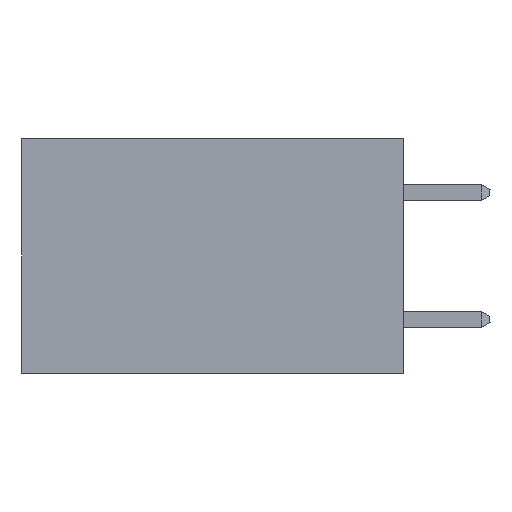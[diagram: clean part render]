
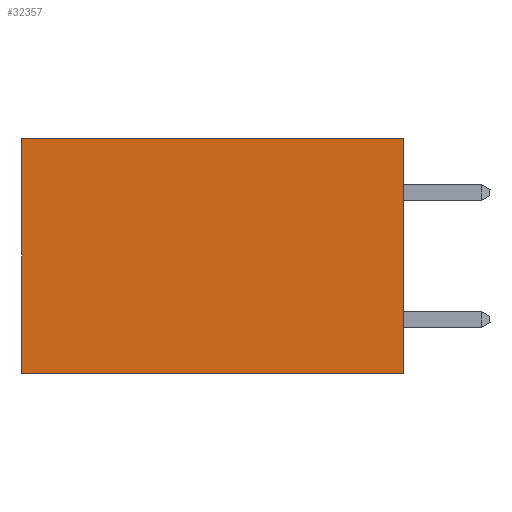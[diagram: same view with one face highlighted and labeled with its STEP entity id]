
A CAD part, left-side view. The second image highlights one B-rep face of the part: STEP entity #32357.
In plain terms, the highlighted planar face has unit normal (-1, 0, 0).
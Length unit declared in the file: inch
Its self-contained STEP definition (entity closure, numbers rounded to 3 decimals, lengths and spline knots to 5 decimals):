
#1623 = CARTESIAN_POINT ( 'NONE',  ( 0.2875, 0., 0. ) ) ;
#1764 = VERTEX_POINT ( 'NONE', #30921 ) ;
#2161 = DIRECTION ( 'NONE',  ( 0., 0., -1. ) ) ;
#2675 = LINE ( 'NONE', #16467, #3827 ) ;
#3013 = PLANE ( 'NONE',  #22933 ) ;
#3535 = ORIENTED_EDGE ( 'NONE', *, *, #15642, .F. ) ;
#3827 = VECTOR ( 'NONE', #2161, 39.37008 ) ;
#7677 = VECTOR ( 'NONE', #17593, 39.37008 ) ;
#7687 = DIRECTION ( 'NONE',  ( 0., 0., -1. ) ) ;
#8514 = FACE_OUTER_BOUND ( 'NONE', #14511, .T. ) ;
#9731 = LINE ( 'NONE', #27854, #22397 ) ;
#10199 = LINE ( 'NONE', #27157, #28822 ) ;
#13163 = ORIENTED_EDGE ( 'NONE', *, *, #20071, .T. ) ;
#14511 = EDGE_LOOP ( 'NONE', ( #13163, #3535, #28302, #31554 ) ) ;
#15642 = EDGE_CURVE ( 'NONE', #30937, #1764, #16727, .T. ) ;
#16467 = CARTESIAN_POINT ( 'NONE',  ( 0.2875, 0.6, 0. ) ) ;
#16727 = LINE ( 'NONE', #27665, #7677 ) ;
#17593 = DIRECTION ( 'NONE',  ( 0., 1., 0. ) ) ;
#17914 = DIRECTION ( 'NONE',  ( 1., 0., 0. ) ) ;
#20071 = EDGE_CURVE ( 'NONE', #31654, #1764, #2675, .T. ) ;
#20657 = CARTESIAN_POINT ( 'NONE',  ( 0.2875, 0., 0. ) ) ;
#22203 = CARTESIAN_POINT ( 'NONE',  ( 0.2875, 0.6, 0. ) ) ;
#22397 = VECTOR ( 'NONE', #32657, 39.37008 ) ;
#22933 = AXIS2_PLACEMENT_3D ( 'NONE', #20657, #17914, #7687 ) ;
#24709 = CARTESIAN_POINT ( 'NONE',  ( 0.2875, 0., -0.37 ) ) ;
#24743 = DIRECTION ( 'NONE',  ( 0., 1., 0. ) ) ;
#24805 = EDGE_CURVE ( 'NONE', #29007, #30937, #9731, .T. ) ;
#27157 = CARTESIAN_POINT ( 'NONE',  ( 0.2875, 0., 0. ) ) ;
#27665 = CARTESIAN_POINT ( 'NONE',  ( 0.2875, 0., -0.37 ) ) ;
#27854 = CARTESIAN_POINT ( 'NONE',  ( 0.2875, 0., 0. ) ) ;
#28302 = ORIENTED_EDGE ( 'NONE', *, *, #24805, .F. ) ;
#28822 = VECTOR ( 'NONE', #24743, 39.37008 ) ;
#29007 = VERTEX_POINT ( 'NONE', #1623 ) ;
#30364 = EDGE_CURVE ( 'NONE', #29007, #31654, #10199, .T. ) ;
#30921 = CARTESIAN_POINT ( 'NONE',  ( 0.2875, 0.6, -0.37 ) ) ;
#30937 = VERTEX_POINT ( 'NONE', #24709 ) ;
#31554 = ORIENTED_EDGE ( 'NONE', *, *, #30364, .T. ) ;
#31654 = VERTEX_POINT ( 'NONE', #22203 ) ;
#32357 = ADVANCED_FACE ( 'NONE', ( #8514 ), #3013, .F. ) ;
#32657 = DIRECTION ( 'NONE',  ( 0., 0., -1. ) ) ;
